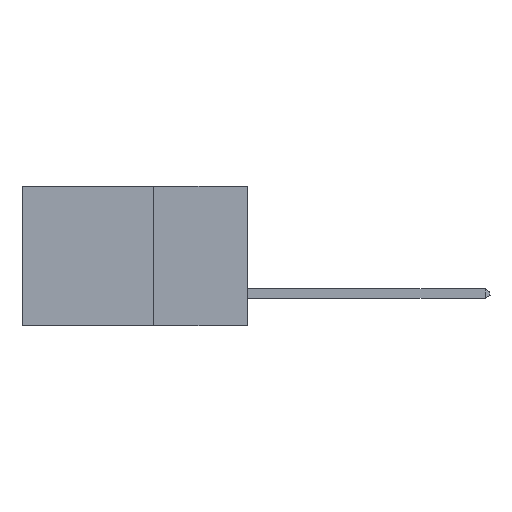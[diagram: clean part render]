
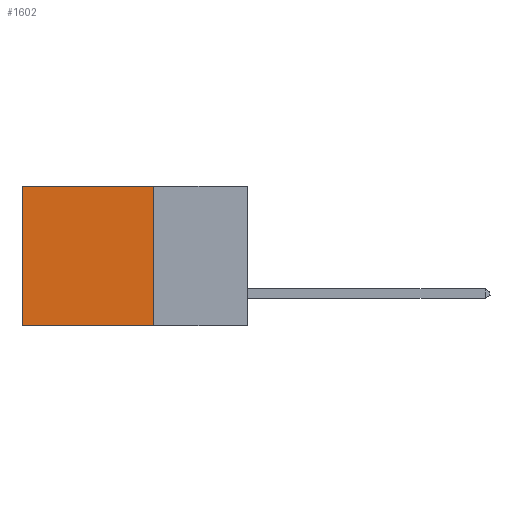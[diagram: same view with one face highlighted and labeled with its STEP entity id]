
A CAD part, left-side view. The second image highlights one B-rep face of the part: STEP entity #1602.
In plain terms, the highlighted planar face has unit normal (-1, 0, 0).
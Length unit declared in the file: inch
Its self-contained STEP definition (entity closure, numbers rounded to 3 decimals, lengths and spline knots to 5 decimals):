
#196 = CARTESIAN_POINT ( 'NONE',  ( 0.298, 0.6, -0.37 ) ) ;
#1471 = EDGE_CURVE ( 'NONE', #10572, #2484, #6266, .T. ) ;
#1587 = LINE ( 'NONE', #2027, #3349 ) ;
#1602 = ADVANCED_FACE ( 'NONE', ( #2472 ), #9719, .F. ) ;
#1858 = DIRECTION ( 'NONE',  ( 0., 1., 0. ) ) ;
#1887 = ORIENTED_EDGE ( 'NONE', *, *, #1471, .F. ) ;
#1894 = LINE ( 'NONE', #7928, #6136 ) ;
#1951 = DIRECTION ( 'NONE',  ( 1., 0., 0. ) ) ;
#2027 = CARTESIAN_POINT ( 'NONE',  ( 0.298, 0.25, 0. ) ) ;
#2472 = FACE_OUTER_BOUND ( 'NONE', #11600, .T. ) ;
#2484 = VERTEX_POINT ( 'NONE', #196 ) ;
#2576 = DIRECTION ( 'NONE',  ( 0., 1., 0. ) ) ;
#3105 = DIRECTION ( 'NONE',  ( 0., 0., -1. ) ) ;
#3349 = VECTOR ( 'NONE', #5585, 39.37008 ) ;
#3483 = VECTOR ( 'NONE', #2576, 39.37008 ) ;
#3581 = VERTEX_POINT ( 'NONE', #10019 ) ;
#3625 = CARTESIAN_POINT ( 'NONE',  ( 0.298, 0.25, -0.37 ) ) ;
#3707 = ORIENTED_EDGE ( 'NONE', *, *, #8983, .F. ) ;
#3818 = CARTESIAN_POINT ( 'NONE',  ( 0.298, 0.25, 0. ) ) ;
#3910 = EDGE_CURVE ( 'NONE', #4077, #2484, #1894, .T. ) ;
#4077 = VERTEX_POINT ( 'NONE', #10996 ) ;
#4659 = CARTESIAN_POINT ( 'NONE',  ( 0.298, 0.25, 0. ) ) ;
#4673 = ORIENTED_EDGE ( 'NONE', *, *, #3910, .T. ) ;
#4729 = DIRECTION ( 'NONE',  ( 0., 0., -1. ) ) ;
#4792 = LINE ( 'NONE', #3818, #11699 ) ;
#5463 = ORIENTED_EDGE ( 'NONE', *, *, #11020, .T. ) ;
#5585 = DIRECTION ( 'NONE',  ( 0., 0., -1. ) ) ;
#6136 = VECTOR ( 'NONE', #3105, 39.37008 ) ;
#6266 = LINE ( 'NONE', #7172, #3483 ) ;
#7172 = CARTESIAN_POINT ( 'NONE',  ( 0.298, 0.25, -0.37 ) ) ;
#7928 = CARTESIAN_POINT ( 'NONE',  ( 0.298, 0.6, 0. ) ) ;
#8983 = EDGE_CURVE ( 'NONE', #3581, #10572, #1587, .T. ) ;
#9719 = PLANE ( 'NONE',  #11670 ) ;
#10019 = CARTESIAN_POINT ( 'NONE',  ( 0.298, 0.25, 0. ) ) ;
#10572 = VERTEX_POINT ( 'NONE', #3625 ) ;
#10996 = CARTESIAN_POINT ( 'NONE',  ( 0.298, 0.6, 0. ) ) ;
#11020 = EDGE_CURVE ( 'NONE', #3581, #4077, #4792, .T. ) ;
#11600 = EDGE_LOOP ( 'NONE', ( #4673, #1887, #3707, #5463 ) ) ;
#11670 = AXIS2_PLACEMENT_3D ( 'NONE', #4659, #1951, #4729 ) ;
#11699 = VECTOR ( 'NONE', #1858, 39.37008 ) ;
